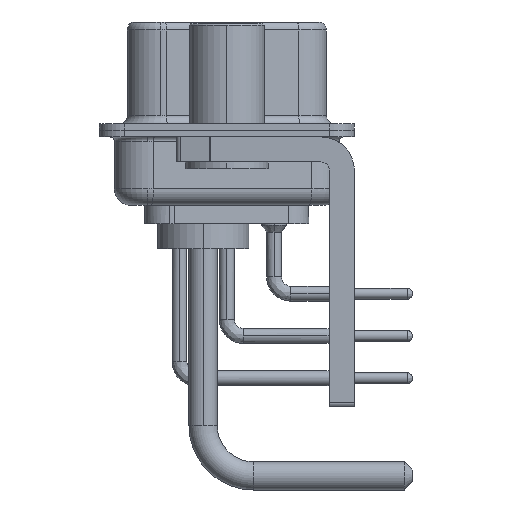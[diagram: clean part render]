
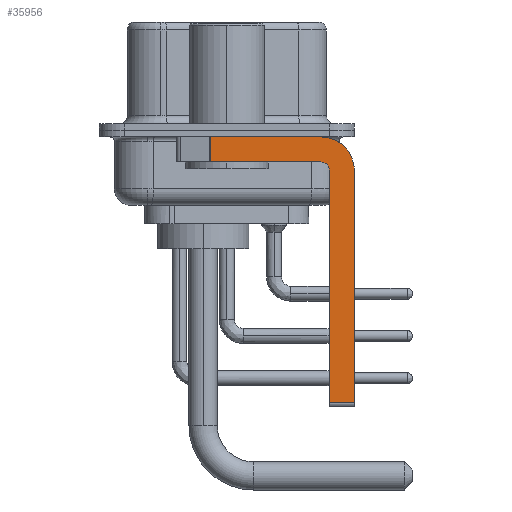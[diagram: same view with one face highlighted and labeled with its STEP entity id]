
A CAD part, left-side view. The second image highlights one B-rep face of the part: STEP entity #35956.
In plain terms, the highlighted planar face has unit normal (-1, 0, 0).
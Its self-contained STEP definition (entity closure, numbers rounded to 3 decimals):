
#190 = CARTESIAN_POINT ( 'NONE',  ( -2.9, -5.65, -2.4 ) ) ;
#280 = DIRECTION ( 'NONE',  ( 0., 1., 0. ) ) ;
#2067 = LINE ( 'NONE', #10417, #7728 ) ;
#2567 = CARTESIAN_POINT ( 'NONE',  ( -2.9, -5.65, -0.4 ) ) ;
#2763 = EDGE_CURVE ( 'NONE', #36300, #20246, #24187, .T. ) ;
#2866 = VECTOR ( 'NONE', #3831, 1000. ) ;
#3165 = VECTOR ( 'NONE', #280, 1000. ) ;
#3831 = DIRECTION ( 'NONE',  ( 0., 0., -1. ) ) ;
#4009 = LINE ( 'NONE', #7351, #2866 ) ;
#4710 = CARTESIAN_POINT ( 'NONE',  ( -2.9, 3., -0.4 ) ) ;
#5230 = ORIENTED_EDGE ( 'NONE', *, *, #2763, .F. ) ;
#5296 = CARTESIAN_POINT ( 'NONE',  ( -2.9, -7.65, -16.35 ) ) ;
#5474 = LINE ( 'NONE', #17192, #3165 ) ;
#5740 = EDGE_CURVE ( 'NONE', #14536, #32116, #19815, .T. ) ;
#5793 = VECTOR ( 'NONE', #10524, 1000. ) ;
#6018 = DIRECTION ( 'NONE',  ( 1., 0., 0. ) ) ;
#6127 = DIRECTION ( 'NONE',  ( 1., 0., 0. ) ) ;
#6303 = FACE_OUTER_BOUND ( 'NONE', #11699, .T. ) ;
#7277 = ORIENTED_EDGE ( 'NONE', *, *, #29425, .F. ) ;
#7351 = CARTESIAN_POINT ( 'NONE',  ( -2.9, 0.978, -1.9 ) ) ;
#7728 = VECTOR ( 'NONE', #32919, 1000. ) ;
#8717 = EDGE_CURVE ( 'NONE', #20246, #21573, #2067, .T. ) ;
#9249 = DIRECTION ( 'NONE',  ( -1., 0., 0. ) ) ;
#9495 = EDGE_CURVE ( 'NONE', #21308, #36300, #10823, .T. ) ;
#10417 = CARTESIAN_POINT ( 'NONE',  ( -2.9, -7.65, -2.4 ) ) ;
#10524 = DIRECTION ( 'NONE',  ( 0., 0., 1. ) ) ;
#10823 = LINE ( 'NONE', #4710, #28563 ) ;
#11545 = CARTESIAN_POINT ( 'NONE',  ( -2.9, -7.65, -2.4 ) ) ;
#11699 = EDGE_LOOP ( 'NONE', ( #26886, #35999, #14034, #7277, #27952, #22100, #36109, #5230 ) ) ;
#13247 = CARTESIAN_POINT ( 'NONE',  ( -2.9, -5.65, -16.35 ) ) ;
#14034 = ORIENTED_EDGE ( 'NONE', *, *, #19708, .F. ) ;
#14308 = DIRECTION ( 'NONE',  ( 0., 0., -1. ) ) ;
#14536 = VERTEX_POINT ( 'NONE', #26762 ) ;
#15713 = CARTESIAN_POINT ( 'NONE',  ( -2.9, -5.65, -2.4 ) ) ;
#17032 = CARTESIAN_POINT ( 'NONE',  ( -2.9, -6.15, -16.6 ) ) ;
#17192 = CARTESIAN_POINT ( 'NONE',  ( -2.9, -5.65, -1.9 ) ) ;
#17364 = DIRECTION ( 'NONE',  ( 0., 0., -1. ) ) ;
#18393 = CARTESIAN_POINT ( 'NONE',  ( -2.9, -6.15, -2.4 ) ) ;
#19074 = VERTEX_POINT ( 'NONE', #22437 ) ;
#19708 = EDGE_CURVE ( 'NONE', #19074, #26274, #5474, .T. ) ;
#19815 = LINE ( 'NONE', #17032, #5793 ) ;
#20246 = VERTEX_POINT ( 'NONE', #11545 ) ;
#20751 = CARTESIAN_POINT ( 'NONE',  ( -2.9, 0.978, -0.4 ) ) ;
#21216 = AXIS2_PLACEMENT_3D ( 'NONE', #31485, #6018, #17364 ) ;
#21308 = VERTEX_POINT ( 'NONE', #20751 ) ;
#21573 = VERTEX_POINT ( 'NONE', #5296 ) ;
#22100 = ORIENTED_EDGE ( 'NONE', *, *, #27058, .T. ) ;
#22437 = CARTESIAN_POINT ( 'NONE',  ( -2.9, -5.65, -1.9 ) ) ;
#24187 = CIRCLE ( 'NONE', #21216, 2. ) ;
#26007 = EDGE_CURVE ( 'NONE', #21308, #26274, #4009, .T. ) ;
#26274 = VERTEX_POINT ( 'NONE', #34958 ) ;
#26762 = CARTESIAN_POINT ( 'NONE',  ( -2.9, -6.15, -16.35 ) ) ;
#26886 = ORIENTED_EDGE ( 'NONE', *, *, #9495, .F. ) ;
#27058 = EDGE_CURVE ( 'NONE', #14536, #21573, #27380, .T. ) ;
#27184 = VECTOR ( 'NONE', #36112, 1000. ) ;
#27380 = LINE ( 'NONE', #13247, #27184 ) ;
#27952 = ORIENTED_EDGE ( 'NONE', *, *, #5740, .F. ) ;
#28563 = VECTOR ( 'NONE', #35933, 1000. ) ;
#29425 = EDGE_CURVE ( 'NONE', #32116, #19074, #34293, .T. ) ;
#30738 = AXIS2_PLACEMENT_3D ( 'NONE', #15713, #9249, #31922 ) ;
#31485 = CARTESIAN_POINT ( 'NONE',  ( -2.9, -5.65, -2.4 ) ) ;
#31605 = AXIS2_PLACEMENT_3D ( 'NONE', #190, #6127, #14308 ) ;
#31922 = DIRECTION ( 'NONE',  ( 0., 0., 1. ) ) ;
#32116 = VERTEX_POINT ( 'NONE', #18393 ) ;
#32919 = DIRECTION ( 'NONE',  ( 0., 0., -1. ) ) ;
#34197 = PLANE ( 'NONE',  #31605 ) ;
#34293 = CIRCLE ( 'NONE', #30738, 0.5 ) ;
#34958 = CARTESIAN_POINT ( 'NONE',  ( -2.9, 0.978, -1.9 ) ) ;
#35933 = DIRECTION ( 'NONE',  ( 0., -1., 0. ) ) ;
#35956 = ADVANCED_FACE ( 'NONE', ( #6303 ), #34197, .F. ) ;
#35999 = ORIENTED_EDGE ( 'NONE', *, *, #26007, .T. ) ;
#36109 = ORIENTED_EDGE ( 'NONE', *, *, #8717, .F. ) ;
#36112 = DIRECTION ( 'NONE',  ( 0., -1., 0. ) ) ;
#36300 = VERTEX_POINT ( 'NONE', #2567 ) ;
